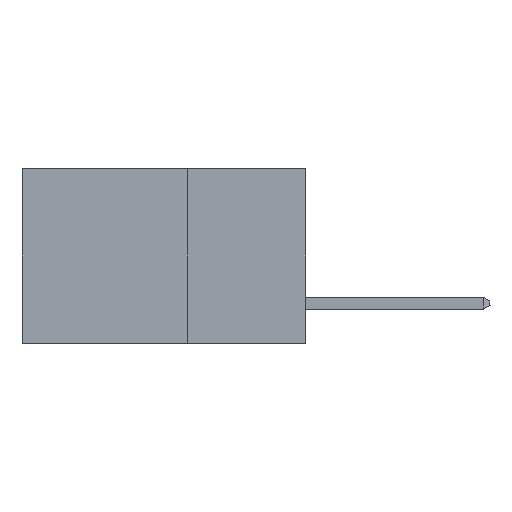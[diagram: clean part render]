
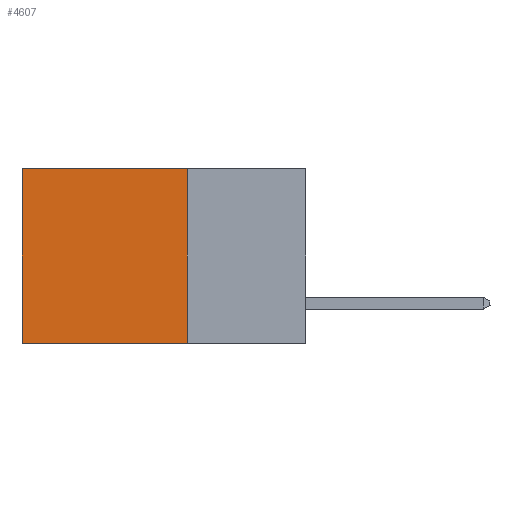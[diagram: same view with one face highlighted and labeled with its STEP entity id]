
A CAD part, left-side view. The second image highlights one B-rep face of the part: STEP entity #4607.
In plain terms, the highlighted planar face has unit normal (-1, 0, 0).
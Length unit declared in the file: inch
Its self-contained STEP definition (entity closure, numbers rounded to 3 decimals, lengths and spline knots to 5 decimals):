
#975 = CARTESIAN_POINT ( 'NONE',  ( 0.298, 0.6, 0. ) ) ;
#1219 = ORIENTED_EDGE ( 'NONE', *, *, #2654, .F. ) ;
#1503 = DIRECTION ( 'NONE',  ( 0., 0., -1. ) ) ;
#2060 = VECTOR ( 'NONE', #10773, 39.37008 ) ;
#2121 = VERTEX_POINT ( 'NONE', #6563 ) ;
#2654 = EDGE_CURVE ( 'NONE', #12552, #7441, #8558, .T. ) ;
#2787 = EDGE_CURVE ( 'NONE', #12552, #10128, #9913, .T. ) ;
#2961 = DIRECTION ( 'NONE',  ( 0., 0., -1. ) ) ;
#3096 = VECTOR ( 'NONE', #9309, 39.37008 ) ;
#3658 = CARTESIAN_POINT ( 'NONE',  ( 0.298, 0.6, 0. ) ) ;
#3775 = CARTESIAN_POINT ( 'NONE',  ( 0.298, 0.25, -0.37 ) ) ;
#4607 = ADVANCED_FACE ( 'NONE', ( #9187 ), #5188, .F. ) ;
#5188 = PLANE ( 'NONE',  #11690 ) ;
#6241 = EDGE_CURVE ( 'NONE', #10128, #2121, #7260, .T. ) ;
#6563 = CARTESIAN_POINT ( 'NONE',  ( 0.298, 0.6, -0.37 ) ) ;
#6834 = VECTOR ( 'NONE', #2961, 39.37008 ) ;
#6870 = ORIENTED_EDGE ( 'NONE', *, *, #8392, .F. ) ;
#7260 = LINE ( 'NONE', #3658, #10345 ) ;
#7286 = DIRECTION ( 'NONE',  ( 0., 0., -1. ) ) ;
#7314 = CARTESIAN_POINT ( 'NONE',  ( 0.298, 0.25, 0. ) ) ;
#7441 = VERTEX_POINT ( 'NONE', #8215 ) ;
#8215 = CARTESIAN_POINT ( 'NONE',  ( 0.298, 0.25, -0.37 ) ) ;
#8392 = EDGE_CURVE ( 'NONE', #7441, #2121, #9926, .T. ) ;
#8490 = CARTESIAN_POINT ( 'NONE',  ( 0.298, 0.25, 0. ) ) ;
#8558 = LINE ( 'NONE', #7314, #6834 ) ;
#8704 = EDGE_LOOP ( 'NONE', ( #10197, #6870, #1219, #10192 ) ) ;
#9187 = FACE_OUTER_BOUND ( 'NONE', #8704, .T. ) ;
#9309 = DIRECTION ( 'NONE',  ( 0., 1., 0. ) ) ;
#9580 = CARTESIAN_POINT ( 'NONE',  ( 0.298, 0.25, 0. ) ) ;
#9913 = LINE ( 'NONE', #12914, #2060 ) ;
#9926 = LINE ( 'NONE', #3775, #3096 ) ;
#10128 = VERTEX_POINT ( 'NONE', #975 ) ;
#10192 = ORIENTED_EDGE ( 'NONE', *, *, #2787, .T. ) ;
#10197 = ORIENTED_EDGE ( 'NONE', *, *, #6241, .T. ) ;
#10345 = VECTOR ( 'NONE', #1503, 39.37008 ) ;
#10773 = DIRECTION ( 'NONE',  ( 0., 1., 0. ) ) ;
#11605 = DIRECTION ( 'NONE',  ( 1., 0., 0. ) ) ;
#11690 = AXIS2_PLACEMENT_3D ( 'NONE', #8490, #11605, #7286 ) ;
#12552 = VERTEX_POINT ( 'NONE', #9580 ) ;
#12914 = CARTESIAN_POINT ( 'NONE',  ( 0.298, 0.25, 0. ) ) ;
